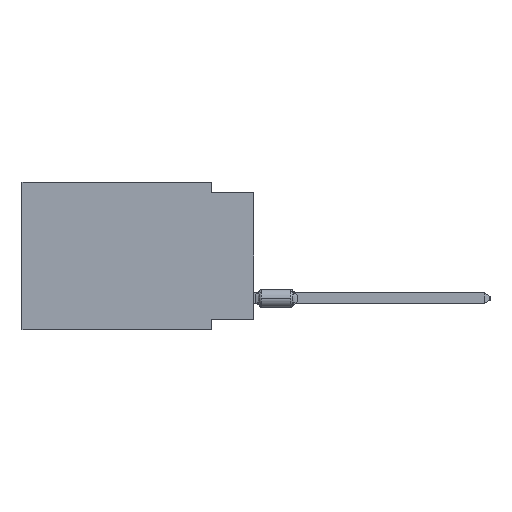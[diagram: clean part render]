
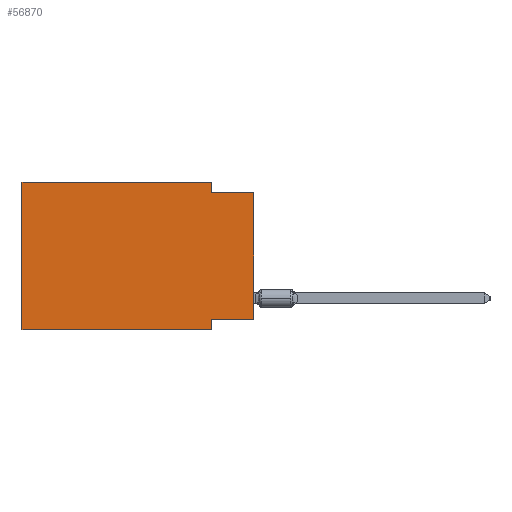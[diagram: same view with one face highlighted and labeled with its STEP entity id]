
A CAD part, left-side view. The second image highlights one B-rep face of the part: STEP entity #56870.
In plain terms, the highlighted planar face has unit normal (-1, 0, 0).
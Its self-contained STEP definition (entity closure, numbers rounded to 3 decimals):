
#1505 = LINE ( 'NONE', #18761, #51643 ) ;
#2029 = CARTESIAN_POINT ( 'NONE',  ( 0., 2.54, -8.89 ) ) ;
#4056 = CARTESIAN_POINT ( 'NONE',  ( 0., 13.97, -8.89 ) ) ;
#4786 = CARTESIAN_POINT ( 'NONE',  ( 0., 13.97, 0. ) ) ;
#6399 = VERTEX_POINT ( 'NONE', #21847 ) ;
#8584 = VECTOR ( 'NONE', #33748, 1000. ) ;
#9057 = VERTEX_POINT ( 'NONE', #20639 ) ;
#10136 = VECTOR ( 'NONE', #67571, 1000. ) ;
#10720 = CARTESIAN_POINT ( 'NONE',  ( 0., 2.54, 0. ) ) ;
#10949 = DIRECTION ( 'NONE',  ( 0., 0., -1. ) ) ;
#12286 = VECTOR ( 'NONE', #27107, 1000. ) ;
#15651 = DIRECTION ( 'NONE',  ( 0., -1., 0. ) ) ;
#15723 = VERTEX_POINT ( 'NONE', #100272 ) ;
#18761 = CARTESIAN_POINT ( 'NONE',  ( 0., 2.54, 0. ) ) ;
#19141 = VERTEX_POINT ( 'NONE', #4056 ) ;
#20639 = CARTESIAN_POINT ( 'NONE',  ( 0., 0., -0.635 ) ) ;
#21847 = CARTESIAN_POINT ( 'NONE',  ( 0., 13.97, 0. ) ) ;
#24119 = ORIENTED_EDGE ( 'NONE', *, *, #58183, .F. ) ;
#24654 = LINE ( 'NONE', #51927, #57819 ) ;
#27107 = DIRECTION ( 'NONE',  ( 0., 0., -1. ) ) ;
#28186 = EDGE_LOOP ( 'NONE', ( #73303, #44571, #24119, #49523, #83106, #64389, #57361, #87366 ) ) ;
#31241 = VECTOR ( 'NONE', #15651, 1000. ) ;
#31272 = VECTOR ( 'NONE', #51587, 1000. ) ;
#32226 = CARTESIAN_POINT ( 'NONE',  ( 0., 0., -8.255 ) ) ;
#33748 = DIRECTION ( 'NONE',  ( 0., 0., 1. ) ) ;
#34104 = LINE ( 'NONE', #59767, #10136 ) ;
#35047 = EDGE_CURVE ( 'NONE', #6399, #37621, #96546, .T. ) ;
#35480 = LINE ( 'NONE', #2029, #12286 ) ;
#37621 = VERTEX_POINT ( 'NONE', #10720 ) ;
#38018 = DIRECTION ( 'NONE',  ( 0., -1., 0. ) ) ;
#44340 = EDGE_CURVE ( 'NONE', #81333, #9057, #74470, .T. ) ;
#44571 = ORIENTED_EDGE ( 'NONE', *, *, #66103, .F. ) ;
#49523 = ORIENTED_EDGE ( 'NONE', *, *, #35047, .F. ) ;
#51587 = DIRECTION ( 'NONE',  ( 0., -1., 0. ) ) ;
#51643 = VECTOR ( 'NONE', #10949, 1000. ) ;
#51927 = CARTESIAN_POINT ( 'NONE',  ( 0., 13.97, 0. ) ) ;
#54936 = PLANE ( 'NONE',  #101219 ) ;
#55469 = EDGE_CURVE ( 'NONE', #67642, #15723, #35480, .T. ) ;
#55470 = FACE_OUTER_BOUND ( 'NONE', #28186, .T. ) ;
#56870 = ADVANCED_FACE ( 'NONE', ( #55470 ), #54936, .F. ) ;
#57361 = ORIENTED_EDGE ( 'NONE', *, *, #55469, .F. ) ;
#57819 = VECTOR ( 'NONE', #67569, 1000. ) ;
#58183 = EDGE_CURVE ( 'NONE', #37621, #74344, #1505, .T. ) ;
#59767 = CARTESIAN_POINT ( 'NONE',  ( 0., 0., -8.255 ) ) ;
#59965 = LINE ( 'NONE', #93951, #31272 ) ;
#64389 = ORIENTED_EDGE ( 'NONE', *, *, #101378, .T. ) ;
#66103 = EDGE_CURVE ( 'NONE', #74344, #9057, #91997, .T. ) ;
#66943 = CARTESIAN_POINT ( 'NONE',  ( 0., 2.54, -0.635 ) ) ;
#67569 = DIRECTION ( 'NONE',  ( 0., 0., 1. ) ) ;
#67571 = DIRECTION ( 'NONE',  ( 0., 1., 0. ) ) ;
#67642 = VERTEX_POINT ( 'NONE', #89275 ) ;
#70394 = CARTESIAN_POINT ( 'NONE',  ( 0., 13.97, 0. ) ) ;
#73303 = ORIENTED_EDGE ( 'NONE', *, *, #44340, .T. ) ;
#73325 = DIRECTION ( 'NONE',  ( 1., 0., 0. ) ) ;
#74344 = VERTEX_POINT ( 'NONE', #66943 ) ;
#74470 = LINE ( 'NONE', #84464, #8584 ) ;
#81333 = VERTEX_POINT ( 'NONE', #32226 ) ;
#83106 = ORIENTED_EDGE ( 'NONE', *, *, #96559, .F. ) ;
#84464 = CARTESIAN_POINT ( 'NONE',  ( 0., 0., 0. ) ) ;
#87366 = ORIENTED_EDGE ( 'NONE', *, *, #102754, .F. ) ;
#89275 = CARTESIAN_POINT ( 'NONE',  ( 0., 2.54, -8.255 ) ) ;
#91997 = LINE ( 'NONE', #100895, #31241 ) ;
#93951 = CARTESIAN_POINT ( 'NONE',  ( 0., 13.97, -8.89 ) ) ;
#96546 = LINE ( 'NONE', #70394, #106799 ) ;
#96559 = EDGE_CURVE ( 'NONE', #19141, #6399, #24654, .T. ) ;
#100272 = CARTESIAN_POINT ( 'NONE',  ( 0., 2.54, -8.89 ) ) ;
#100895 = CARTESIAN_POINT ( 'NONE',  ( 0., 0., -0.635 ) ) ;
#101219 = AXIS2_PLACEMENT_3D ( 'NONE', #4786, #73325, #107303 ) ;
#101378 = EDGE_CURVE ( 'NONE', #19141, #15723, #59965, .T. ) ;
#102754 = EDGE_CURVE ( 'NONE', #81333, #67642, #34104, .T. ) ;
#106799 = VECTOR ( 'NONE', #38018, 1000. ) ;
#107303 = DIRECTION ( 'NONE',  ( 0., 0., -1. ) ) ;
